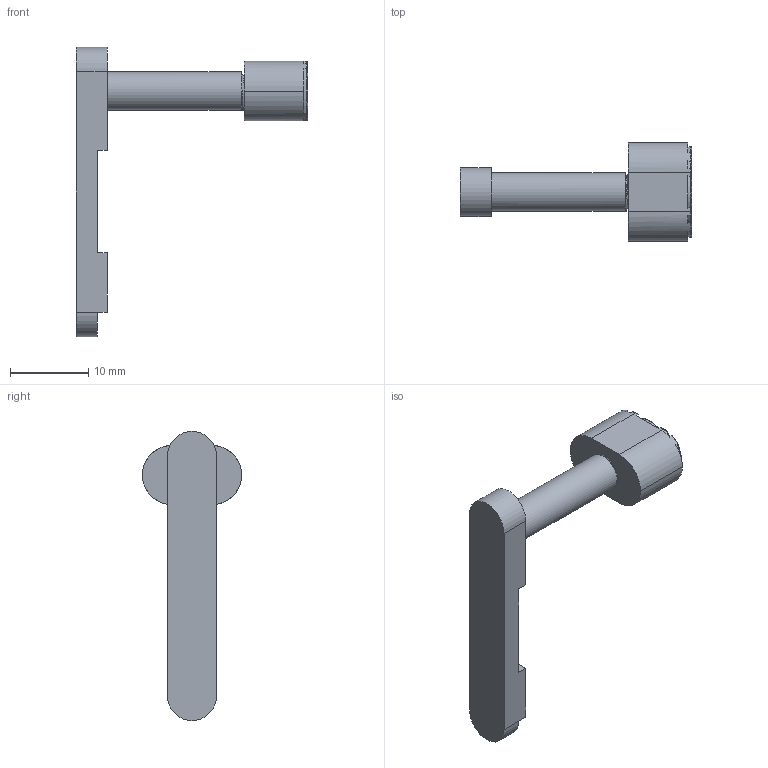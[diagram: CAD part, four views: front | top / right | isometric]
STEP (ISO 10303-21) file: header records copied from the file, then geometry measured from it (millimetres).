
FILE_DESCRIPTION(/* description */ (''),/* implementation_level */ '2;1');
FILE_NAME(/* name */ 'SVTR_Mag Release',/* author */ ('Gunny McGunsmith'),/* organization */ ('AWCY?'),/* authorisation */ '');
FILE_SCHEMA (('AUTOMOTIVE_DESIGN { 1 0 10303 214 3 1 1 }'));
Length unit declared in the file: millimetre
Products named in the file (1): SVTR_Mag Release
Bounding box: 29.61 x 12.7 x 37.05 mm (x, y, z)
Volume: 1732 mm3; surface area: 1817 mm2
Topology: 2 solids, 2 shells, 112 faces, 360 edges, 254 vertices
Faces by surface type: cylinder 62, plane 28, torus 18, bspline 4
Full cylindrical faces by diameter (mm): 3.99 x9, 4.234 x8, 4.901 x11, 5.12 x8, 6.62 x1, 7.62 x1
Entity records: 17617 total; most frequent: CARTESIAN_POINT 14886, ORIENTED_EDGE 654, DIRECTION 454, EDGE_CURVE 327, VERTEX_POINT 232, AXIS2_PLACEMENT_3D 182, B_SPLINE_CURVE_WITH_KNOTS 154, EDGE_LOOP 107
